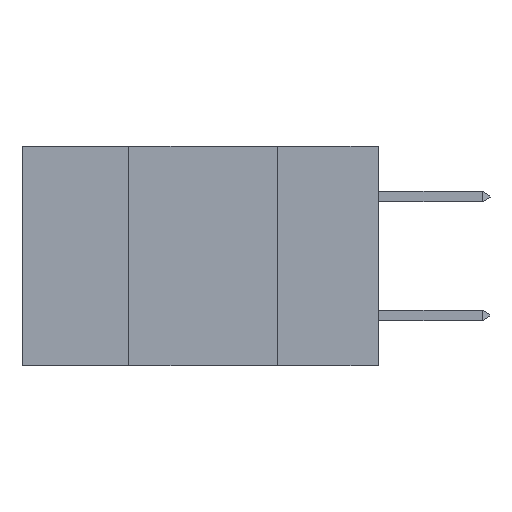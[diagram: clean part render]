
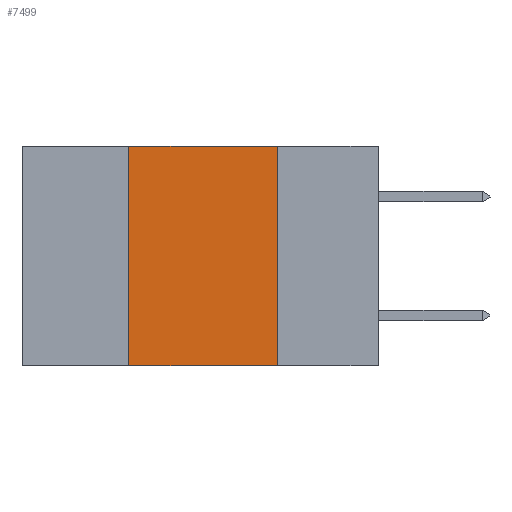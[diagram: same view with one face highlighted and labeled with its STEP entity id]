
A CAD part, left-side view. The second image highlights one B-rep face of the part: STEP entity #7499.
In plain terms, the highlighted planar face has unit normal (-1, 0, 0).
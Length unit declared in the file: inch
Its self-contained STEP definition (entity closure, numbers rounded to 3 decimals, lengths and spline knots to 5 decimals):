
#54 = ORIENTED_EDGE ( 'NONE', *, *, #9463, .F. ) ;
#121 = EDGE_LOOP ( 'NONE', ( #54, #3475, #564, #10080 ) ) ;
#564 = ORIENTED_EDGE ( 'NONE', *, *, #3853, .F. ) ;
#685 = CARTESIAN_POINT ( 'NONE',  ( 0., 0.42, 0. ) ) ;
#2139 = CARTESIAN_POINT ( 'NONE',  ( 0., 0.6, 0. ) ) ;
#2149 = VERTEX_POINT ( 'NONE', #6569 ) ;
#2962 = DIRECTION ( 'NONE',  ( 0., -1., 0. ) ) ;
#3109 = VECTOR ( 'NONE', #8536, 39.37008 ) ;
#3475 = ORIENTED_EDGE ( 'NONE', *, *, #4793, .F. ) ;
#3483 = DIRECTION ( 'NONE',  ( 0., 0., 1. ) ) ;
#3694 = FACE_OUTER_BOUND ( 'NONE', #121, .T. ) ;
#3724 = VECTOR ( 'NONE', #6174, 39.37008 ) ;
#3853 = EDGE_CURVE ( 'NONE', #8110, #8757, #5737, .T. ) ;
#4031 = CARTESIAN_POINT ( 'NONE',  ( 0., 0.17, 0. ) ) ;
#4131 = VECTOR ( 'NONE', #3483, 39.37008 ) ;
#4639 = CARTESIAN_POINT ( 'NONE',  ( 0., 0.17, 0. ) ) ;
#4707 = LINE ( 'NONE', #5416, #6946 ) ;
#4793 = EDGE_CURVE ( 'NONE', #8757, #7597, #4707, .T. ) ;
#5416 = CARTESIAN_POINT ( 'NONE',  ( 0., 0.6, 0. ) ) ;
#5498 = EDGE_CURVE ( 'NONE', #8110, #2149, #6408, .T. ) ;
#5693 = CARTESIAN_POINT ( 'NONE',  ( 0., 0.42, -0.37 ) ) ;
#5737 = LINE ( 'NONE', #6556, #4131 ) ;
#6174 = DIRECTION ( 'NONE',  ( 0., 0., -1. ) ) ;
#6408 = LINE ( 'NONE', #8411, #3109 ) ;
#6556 = CARTESIAN_POINT ( 'NONE',  ( 0., 0.42, 0. ) ) ;
#6569 = CARTESIAN_POINT ( 'NONE',  ( 0., 0.17, -0.37 ) ) ;
#6946 = VECTOR ( 'NONE', #2962, 39.37008 ) ;
#7499 = ADVANCED_FACE ( 'NONE', ( #3694 ), #7728, .F. ) ;
#7597 = VERTEX_POINT ( 'NONE', #4031 ) ;
#7728 = PLANE ( 'NONE',  #8816 ) ;
#8110 = VERTEX_POINT ( 'NONE', #5693 ) ;
#8411 = CARTESIAN_POINT ( 'NONE',  ( 0., 0.6, -0.37 ) ) ;
#8445 = DIRECTION ( 'NONE',  ( 1., 0., 0. ) ) ;
#8536 = DIRECTION ( 'NONE',  ( 0., -1., 0. ) ) ;
#8757 = VERTEX_POINT ( 'NONE', #685 ) ;
#8816 = AXIS2_PLACEMENT_3D ( 'NONE', #2139, #8445, #9241 ) ;
#9241 = DIRECTION ( 'NONE',  ( 0., 0., -1. ) ) ;
#9463 = EDGE_CURVE ( 'NONE', #7597, #2149, #9507, .T. ) ;
#9507 = LINE ( 'NONE', #4639, #3724 ) ;
#10080 = ORIENTED_EDGE ( 'NONE', *, *, #5498, .T. ) ;
